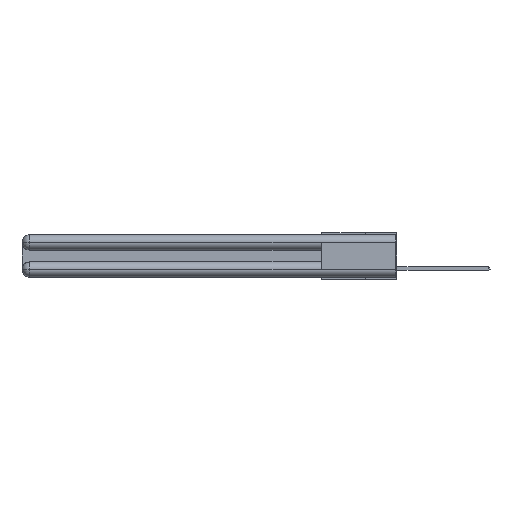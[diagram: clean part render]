
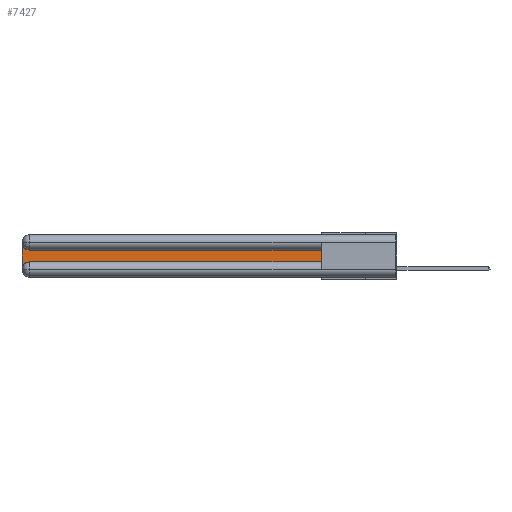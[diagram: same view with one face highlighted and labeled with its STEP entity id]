
A CAD part, left-side view. The second image highlights one B-rep face of the part: STEP entity #7427.
In plain terms, the highlighted planar face has unit normal (-1, 0, 0).
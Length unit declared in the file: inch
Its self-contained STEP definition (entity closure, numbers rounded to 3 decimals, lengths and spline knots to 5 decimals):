
#435 = CARTESIAN_POINT ( 'NONE',  ( 0.075, 3., -0.2175 ) ) ;
#774 = CARTESIAN_POINT ( 'NONE',  ( 0.075, 0.6, -0.2175 ) ) ;
#1121 = EDGE_CURVE ( 'NONE', #11335, #14741, #5436, .T. ) ;
#1239 = AXIS2_PLACEMENT_3D ( 'NONE', #29340, #2045, #14759 ) ;
#1519 = VECTOR ( 'NONE', #19500, 39.37008 ) ;
#1599 = DIRECTION ( 'NONE',  ( 0., 0., -1. ) ) ;
#2045 = DIRECTION ( 'NONE',  ( 1., 0., 0. ) ) ;
#2138 = CIRCLE ( 'NONE', #11517, 0.06 ) ;
#2773 = CARTESIAN_POINT ( 'NONE',  ( 0.075, 3., -0.2775 ) ) ;
#2951 = ORIENTED_EDGE ( 'NONE', *, *, #15133, .T. ) ;
#3357 = AXIS2_PLACEMENT_3D ( 'NONE', #24222, #24326, #29294 ) ;
#3476 = CARTESIAN_POINT ( 'NONE',  ( 0.075, 2.94, -0.1225 ) ) ;
#3837 = CARTESIAN_POINT ( 'NONE',  ( 0.075, 2.94, -0.0625 ) ) ;
#5436 = CIRCLE ( 'NONE', #1239, 0.06 ) ;
#5683 = EDGE_CURVE ( 'NONE', #14741, #22115, #14793, .T. ) ;
#6811 = PLANE ( 'NONE',  #3357 ) ;
#7427 = ADVANCED_FACE ( 'NONE', ( #12398 ), #6811, .F. ) ;
#7434 = LINE ( 'NONE', #15817, #24163 ) ;
#8674 = LINE ( 'NONE', #435, #26601 ) ;
#10226 = ORIENTED_EDGE ( 'NONE', *, *, #13625, .T. ) ;
#10340 = ORIENTED_EDGE ( 'NONE', *, *, #27998, .T. ) ;
#10539 = ORIENTED_EDGE ( 'NONE', *, *, #10697, .T. ) ;
#10697 = EDGE_CURVE ( 'NONE', #24393, #11335, #8674, .T. ) ;
#11335 = VERTEX_POINT ( 'NONE', #2773 ) ;
#11517 = AXIS2_PLACEMENT_3D ( 'NONE', #3837, #31245, #1599 ) ;
#12398 = FACE_OUTER_BOUND ( 'NONE', #16283, .T. ) ;
#12571 = DIRECTION ( 'NONE',  ( 0., -1., 0. ) ) ;
#12996 = ORIENTED_EDGE ( 'NONE', *, *, #1121, .T. ) ;
#13625 = EDGE_CURVE ( 'NONE', #22115, #21039, #20904, .T. ) ;
#14741 = VERTEX_POINT ( 'NONE', #15325 ) ;
#14759 = DIRECTION ( 'NONE',  ( 0., 0., -1. ) ) ;
#14793 = LINE ( 'NONE', #19984, #20319 ) ;
#15133 = EDGE_CURVE ( 'NONE', #27590, #24393, #2138, .T. ) ;
#15325 = CARTESIAN_POINT ( 'NONE',  ( 0.075, 2.94, -0.2175 ) ) ;
#15817 = CARTESIAN_POINT ( 'NONE',  ( 0.075, 0.6, -0.1225 ) ) ;
#16283 = EDGE_LOOP ( 'NONE', ( #10340, #2951, #10539, #12996, #18499, #10226 ) ) ;
#17955 = CARTESIAN_POINT ( 'NONE',  ( 0.075, 3., -0.0625 ) ) ;
#18499 = ORIENTED_EDGE ( 'NONE', *, *, #5683, .T. ) ;
#19500 = DIRECTION ( 'NONE',  ( 0., 0., 1. ) ) ;
#19984 = CARTESIAN_POINT ( 'NONE',  ( 0.075, 0.6, -0.2175 ) ) ;
#20260 = CARTESIAN_POINT ( 'NONE',  ( 0.075, 0.6, -0.1225 ) ) ;
#20319 = VECTOR ( 'NONE', #12571, 39.37008 ) ;
#20904 = LINE ( 'NONE', #31734, #1519 ) ;
#21039 = VERTEX_POINT ( 'NONE', #20260 ) ;
#22115 = VERTEX_POINT ( 'NONE', #774 ) ;
#23151 = DIRECTION ( 'NONE',  ( 0., 1., 0. ) ) ;
#24163 = VECTOR ( 'NONE', #23151, 39.37008 ) ;
#24222 = CARTESIAN_POINT ( 'NONE',  ( 0.075, 3., -0.1225 ) ) ;
#24326 = DIRECTION ( 'NONE',  ( 1., 0., 0. ) ) ;
#24393 = VERTEX_POINT ( 'NONE', #17955 ) ;
#26601 = VECTOR ( 'NONE', #27475, 39.37008 ) ;
#27475 = DIRECTION ( 'NONE',  ( 0., 0., -1. ) ) ;
#27590 = VERTEX_POINT ( 'NONE', #3476 ) ;
#27998 = EDGE_CURVE ( 'NONE', #21039, #27590, #7434, .T. ) ;
#29294 = DIRECTION ( 'NONE',  ( 0., 0., -1. ) ) ;
#29340 = CARTESIAN_POINT ( 'NONE',  ( 0.075, 2.94, -0.2775 ) ) ;
#31245 = DIRECTION ( 'NONE',  ( 1., 0., 0. ) ) ;
#31734 = CARTESIAN_POINT ( 'NONE',  ( 0.075, 0.6, -0.2175 ) ) ;
